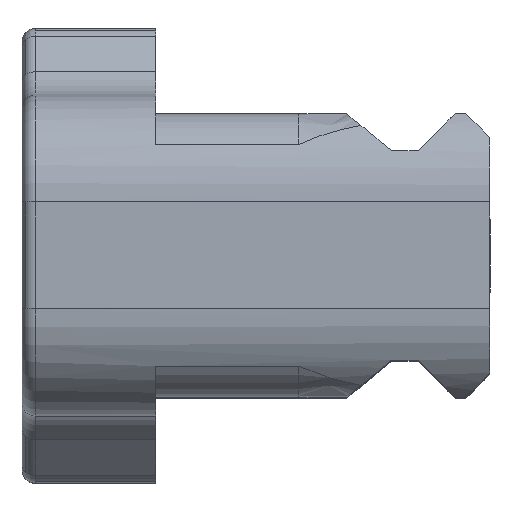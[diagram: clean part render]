
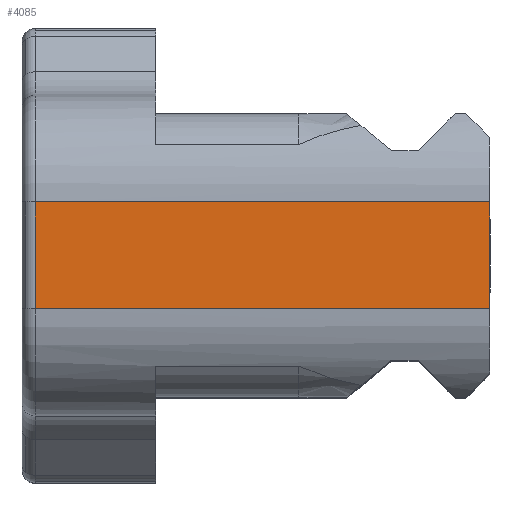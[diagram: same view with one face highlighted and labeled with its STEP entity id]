
A CAD part, top view. The second image highlights one B-rep face of the part: STEP entity #4085.
In plain terms, the highlighted planar face has unit normal (0, 0, 1).
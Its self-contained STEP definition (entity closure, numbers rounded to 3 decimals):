
#362 = AXIS2_PLACEMENT_3D ( 'NONE', #4959, #7201, #3272 ) ;
#371 = VECTOR ( 'NONE', #6392, 1000. ) ;
#600 = LINE ( 'NONE', #3367, #2383 ) ;
#1718 = VERTEX_POINT ( 'NONE', #6827 ) ;
#2030 = VECTOR ( 'NONE', #7018, 1000. ) ;
#2383 = VECTOR ( 'NONE', #6160, 1000. ) ;
#2460 = EDGE_CURVE ( 'NONE', #6596, #1718, #4151, .T. ) ;
#2465 = CARTESIAN_POINT ( 'NONE',  ( 165.981, 0., -71. ) ) ;
#2599 = EDGE_CURVE ( 'NONE', #6541, #6596, #5429, .T. ) ;
#2693 = EDGE_CURVE ( 'NONE', #5978, #1718, #600, .T. ) ;
#2847 = CARTESIAN_POINT ( 'NONE',  ( 165.981, 4., -71. ) ) ;
#3272 = DIRECTION ( 'NONE',  ( 1., 0., 0. ) ) ;
#3284 = EDGE_LOOP ( 'NONE', ( #5822, #4806, #5363, #4935 ) ) ;
#3304 = PLANE ( 'NONE',  #362 ) ;
#3367 = CARTESIAN_POINT ( 'NONE',  ( 130.981, -4., -71. ) ) ;
#3405 = DIRECTION ( 'NONE',  ( 0., 1., 0. ) ) ;
#3712 = CARTESIAN_POINT ( 'NONE',  ( 130.981, 4., -71. ) ) ;
#4085 = ADVANCED_FACE ( 'NONE', ( #7097 ), #3304, .T. ) ;
#4151 = LINE ( 'NONE', #2465, #371 ) ;
#4579 = CARTESIAN_POINT ( 'NONE',  ( 131.981, 2., -71. ) ) ;
#4653 = EDGE_CURVE ( 'NONE', #5978, #6541, #6674, .T. ) ;
#4697 = CARTESIAN_POINT ( 'NONE',  ( 131.981, -4., -71. ) ) ;
#4806 = ORIENTED_EDGE ( 'NONE', *, *, #2599, .F. ) ;
#4935 = ORIENTED_EDGE ( 'NONE', *, *, #2693, .T. ) ;
#4959 = CARTESIAN_POINT ( 'NONE',  ( 130.981, 4., -71. ) ) ;
#5012 = CARTESIAN_POINT ( 'NONE',  ( 131.981, 4., -71. ) ) ;
#5363 = ORIENTED_EDGE ( 'NONE', *, *, #4653, .F. ) ;
#5429 = LINE ( 'NONE', #3712, #2030 ) ;
#5822 = ORIENTED_EDGE ( 'NONE', *, *, #2460, .F. ) ;
#5978 = VERTEX_POINT ( 'NONE', #4697 ) ;
#6160 = DIRECTION ( 'NONE',  ( 1., 0., 0. ) ) ;
#6392 = DIRECTION ( 'NONE',  ( 0., -1., 0. ) ) ;
#6509 = VECTOR ( 'NONE', #3405, 1000. ) ;
#6541 = VERTEX_POINT ( 'NONE', #5012 ) ;
#6596 = VERTEX_POINT ( 'NONE', #2847 ) ;
#6674 = LINE ( 'NONE', #4579, #6509 ) ;
#6827 = CARTESIAN_POINT ( 'NONE',  ( 165.981, -4., -71. ) ) ;
#7018 = DIRECTION ( 'NONE',  ( 1., 0., 0. ) ) ;
#7097 = FACE_OUTER_BOUND ( 'NONE', #3284, .T. ) ;
#7201 = DIRECTION ( 'NONE',  ( 0., 0., 1. ) ) ;
